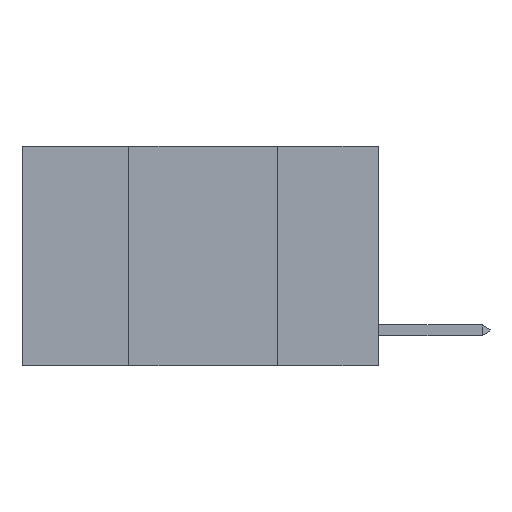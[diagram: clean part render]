
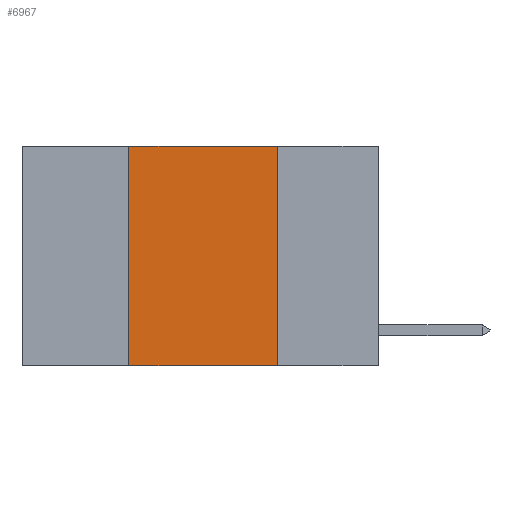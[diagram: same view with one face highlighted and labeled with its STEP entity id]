
A CAD part, left-side view. The second image highlights one B-rep face of the part: STEP entity #6967.
In plain terms, the highlighted planar face has unit normal (-1, 0, 0).
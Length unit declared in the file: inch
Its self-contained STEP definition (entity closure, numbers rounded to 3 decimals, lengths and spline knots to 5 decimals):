
#5 = CARTESIAN_POINT ( 'NONE',  ( 0., 0.42, 0. ) ) ;
#216 = VECTOR ( 'NONE', #5105, 39.37008 ) ;
#679 = VERTEX_POINT ( 'NONE', #2981 ) ;
#1071 = LINE ( 'NONE', #3314, #216 ) ;
#1870 = DIRECTION ( 'NONE',  ( 0., 0., -1. ) ) ;
#2050 = VECTOR ( 'NONE', #1870, 39.37008 ) ;
#2249 = EDGE_LOOP ( 'NONE', ( #5712, #6587, #5286, #3967 ) ) ;
#2798 = DIRECTION ( 'NONE',  ( 0., -1., 0. ) ) ;
#2856 = VERTEX_POINT ( 'NONE', #6593 ) ;
#2981 = CARTESIAN_POINT ( 'NONE',  ( 0., 0.17, 0. ) ) ;
#3314 = CARTESIAN_POINT ( 'NONE',  ( 0., 0.6, -0.37 ) ) ;
#3397 = CARTESIAN_POINT ( 'NONE',  ( 0., 0.42, -0.37 ) ) ;
#3497 = LINE ( 'NONE', #8054, #8210 ) ;
#3611 = LINE ( 'NONE', #5913, #9532 ) ;
#3701 = DIRECTION ( 'NONE',  ( 0., 0., -1. ) ) ;
#3967 = ORIENTED_EDGE ( 'NONE', *, *, #7577, .T. ) ;
#4132 = CARTESIAN_POINT ( 'NONE',  ( 0., 0.17, 0. ) ) ;
#4431 = FACE_OUTER_BOUND ( 'NONE', #2249, .T. ) ;
#4477 = PLANE ( 'NONE',  #6487 ) ;
#4849 = LINE ( 'NONE', #4132, #2050 ) ;
#5105 = DIRECTION ( 'NONE',  ( 0., -1., 0. ) ) ;
#5286 = ORIENTED_EDGE ( 'NONE', *, *, #5313, .F. ) ;
#5313 = EDGE_CURVE ( 'NONE', #6755, #8016, #3497, .T. ) ;
#5712 = ORIENTED_EDGE ( 'NONE', *, *, #5834, .F. ) ;
#5834 = EDGE_CURVE ( 'NONE', #679, #2856, #4849, .T. ) ;
#5913 = CARTESIAN_POINT ( 'NONE',  ( 0., 0.6, 0. ) ) ;
#6487 = AXIS2_PLACEMENT_3D ( 'NONE', #6765, #7477, #3701 ) ;
#6587 = ORIENTED_EDGE ( 'NONE', *, *, #9454, .F. ) ;
#6593 = CARTESIAN_POINT ( 'NONE',  ( 0., 0.17, -0.37 ) ) ;
#6755 = VERTEX_POINT ( 'NONE', #3397 ) ;
#6765 = CARTESIAN_POINT ( 'NONE',  ( 0., 0.6, 0. ) ) ;
#6967 = ADVANCED_FACE ( 'NONE', ( #4431 ), #4477, .F. ) ;
#7477 = DIRECTION ( 'NONE',  ( 1., 0., 0. ) ) ;
#7577 = EDGE_CURVE ( 'NONE', #6755, #2856, #1071, .T. ) ;
#8016 = VERTEX_POINT ( 'NONE', #5 ) ;
#8054 = CARTESIAN_POINT ( 'NONE',  ( 0., 0.42, 0. ) ) ;
#8210 = VECTOR ( 'NONE', #8689, 39.37008 ) ;
#8689 = DIRECTION ( 'NONE',  ( 0., 0., 1. ) ) ;
#9454 = EDGE_CURVE ( 'NONE', #8016, #679, #3611, .T. ) ;
#9532 = VECTOR ( 'NONE', #2798, 39.37008 ) ;
